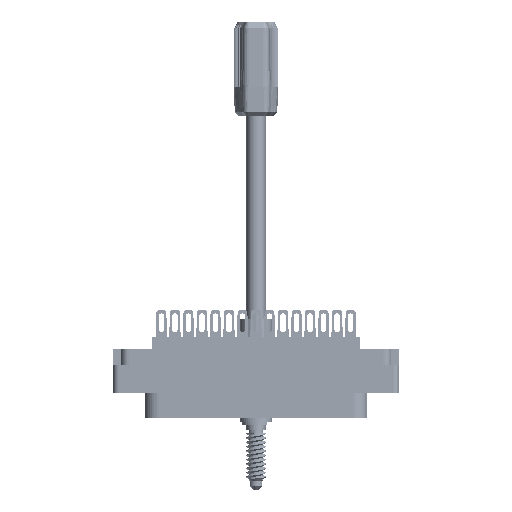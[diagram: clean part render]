
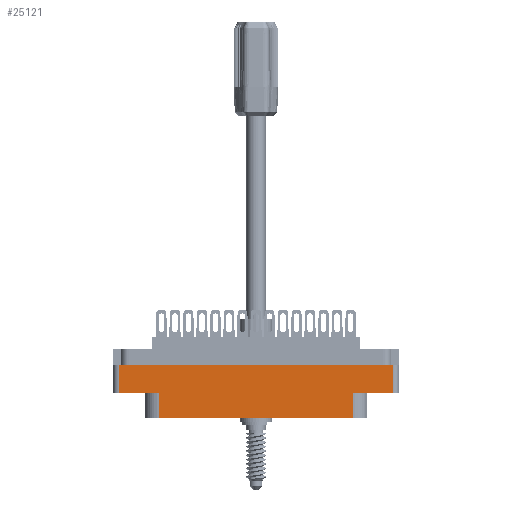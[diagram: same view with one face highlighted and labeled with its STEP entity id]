
A CAD part, front view. The second image highlights one B-rep face of the part: STEP entity #25121.
In plain terms, the highlighted planar face has unit normal (0, -1, 0).
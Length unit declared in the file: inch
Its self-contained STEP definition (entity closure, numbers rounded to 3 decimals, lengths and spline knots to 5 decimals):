
#4005 = EDGE_CURVE ( 'NONE', #22299, #32791, #96610, .T. ) ;
#8165 = EDGE_CURVE ( 'NONE', #33444, #86296, #30305, .T. ) ;
#10724 = DIRECTION ( 'NONE',  ( 1., 0., 0. ) ) ;
#11108 = VECTOR ( 'NONE', #83705, 39.37008 ) ;
#12133 = PLANE ( 'NONE',  #48868 ) ;
#14208 = ORIENTED_EDGE ( 'NONE', *, *, #4005, .F. ) ;
#14694 = CARTESIAN_POINT ( 'NONE',  ( 0., -0.7625, -0.54 ) ) ;
#15535 = VERTEX_POINT ( 'NONE', #22653 ) ;
#22299 = VERTEX_POINT ( 'NONE', #34164 ) ;
#22653 = CARTESIAN_POINT ( 'NONE',  ( -0.9315, -0.7625, -0.54 ) ) ;
#22939 = CARTESIAN_POINT ( 'NONE',  ( 0.9315, -0.7625, -0.54 ) ) ;
#23843 = EDGE_LOOP ( 'NONE', ( #28669, #99431, #40305, #32892, #38980, #90521, #14208, #86673 ) ) ;
#24555 = LINE ( 'NONE', #22939, #55815 ) ;
#25121 = ADVANCED_FACE ( 'NONE', ( #70575 ), #12133, .T. ) ;
#25228 = LINE ( 'NONE', #71312, #39011 ) ;
#26719 = CARTESIAN_POINT ( 'NONE',  ( 0., -0.7625, -0.54 ) ) ;
#27524 = CARTESIAN_POINT ( 'NONE',  ( -1.313, -0.7625, -0.78 ) ) ;
#28084 = EDGE_CURVE ( 'NONE', #44377, #45847, #38636, .T. ) ;
#28669 = ORIENTED_EDGE ( 'NONE', *, *, #28084, .F. ) ;
#30305 = LINE ( 'NONE', #91447, #66603 ) ;
#32791 = VERTEX_POINT ( 'NONE', #42938 ) ;
#32892 = ORIENTED_EDGE ( 'NONE', *, *, #41973, .T. ) ;
#32929 = VECTOR ( 'NONE', #34800, 39.37008 ) ;
#33444 = VERTEX_POINT ( 'NONE', #78133 ) ;
#34164 = CARTESIAN_POINT ( 'NONE',  ( 1.313, -0.7625, -0.54 ) ) ;
#34800 = DIRECTION ( 'NONE',  ( -1., 0., 0. ) ) ;
#38463 = DIRECTION ( 'NONE',  ( 1., 0., 0. ) ) ;
#38636 = LINE ( 'NONE', #83397, #11108 ) ;
#38980 = ORIENTED_EDGE ( 'NONE', *, *, #8165, .T. ) ;
#39011 = VECTOR ( 'NONE', #47908, 39.37008 ) ;
#40305 = ORIENTED_EDGE ( 'NONE', *, *, #99226, .T. ) ;
#40688 = CARTESIAN_POINT ( 'NONE',  ( -1.313, -0.7625, -0.54 ) ) ;
#41973 = EDGE_CURVE ( 'NONE', #15535, #33444, #25228, .T. ) ;
#42917 = CARTESIAN_POINT ( 'NONE',  ( -1.375, -0.7625, -0.78 ) ) ;
#42938 = CARTESIAN_POINT ( 'NONE',  ( 0.9315, -0.7625, -0.54 ) ) ;
#44377 = VERTEX_POINT ( 'NONE', #87967 ) ;
#44682 = DIRECTION ( 'NONE',  ( 0., 0., -1. ) ) ;
#45847 = VERTEX_POINT ( 'NONE', #70256 ) ;
#46506 = LINE ( 'NONE', #14694, #85249 ) ;
#47908 = DIRECTION ( 'NONE',  ( 0., 0., -1. ) ) ;
#48868 = AXIS2_PLACEMENT_3D ( 'NONE', #42917, #76154, #75113 ) ;
#48982 = VECTOR ( 'NONE', #98386, 39.37008 ) ;
#55815 = VECTOR ( 'NONE', #63173, 39.37008 ) ;
#57949 = CARTESIAN_POINT ( 'NONE',  ( 1.313, -0.7625, -0.78 ) ) ;
#63173 = DIRECTION ( 'NONE',  ( 0., 0., 1. ) ) ;
#66603 = VECTOR ( 'NONE', #10724, 39.37008 ) ;
#69725 = CARTESIAN_POINT ( 'NONE',  ( 0.9315, -0.7625, -0.78 ) ) ;
#70256 = CARTESIAN_POINT ( 'NONE',  ( 1.313, -0.7625, -0.274 ) ) ;
#70575 = FACE_OUTER_BOUND ( 'NONE', #23843, .T. ) ;
#71312 = CARTESIAN_POINT ( 'NONE',  ( -0.9315, -0.7625, -0.78 ) ) ;
#75113 = DIRECTION ( 'NONE',  ( 0., 0., -1. ) ) ;
#76154 = DIRECTION ( 'NONE',  ( 0., -1., 0. ) ) ;
#78133 = CARTESIAN_POINT ( 'NONE',  ( -0.9315, -0.7625, -0.78 ) ) ;
#79971 = LINE ( 'NONE', #27524, #96130 ) ;
#82719 = LINE ( 'NONE', #57949, #48982 ) ;
#83397 = CARTESIAN_POINT ( 'NONE',  ( 0., -0.7625, -0.274 ) ) ;
#83567 = VERTEX_POINT ( 'NONE', #40688 ) ;
#83705 = DIRECTION ( 'NONE',  ( 1., 0., 0. ) ) ;
#85249 = VECTOR ( 'NONE', #38463, 39.37008 ) ;
#85654 = EDGE_CURVE ( 'NONE', #44377, #83567, #79971, .T. ) ;
#86296 = VERTEX_POINT ( 'NONE', #69725 ) ;
#86673 = ORIENTED_EDGE ( 'NONE', *, *, #93401, .T. ) ;
#87518 = EDGE_CURVE ( 'NONE', #86296, #32791, #24555, .T. ) ;
#87967 = CARTESIAN_POINT ( 'NONE',  ( -1.313, -0.7625, -0.274 ) ) ;
#90521 = ORIENTED_EDGE ( 'NONE', *, *, #87518, .T. ) ;
#91447 = CARTESIAN_POINT ( 'NONE',  ( -1.375, -0.7625, -0.78 ) ) ;
#93401 = EDGE_CURVE ( 'NONE', #22299, #45847, #82719, .T. ) ;
#96130 = VECTOR ( 'NONE', #44682, 39.37008 ) ;
#96610 = LINE ( 'NONE', #26719, #32929 ) ;
#98386 = DIRECTION ( 'NONE',  ( 0., 0., 1. ) ) ;
#99226 = EDGE_CURVE ( 'NONE', #83567, #15535, #46506, .T. ) ;
#99431 = ORIENTED_EDGE ( 'NONE', *, *, #85654, .T. ) ;
